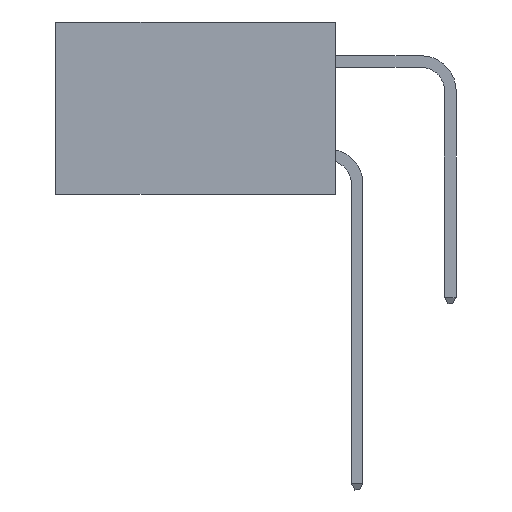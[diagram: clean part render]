
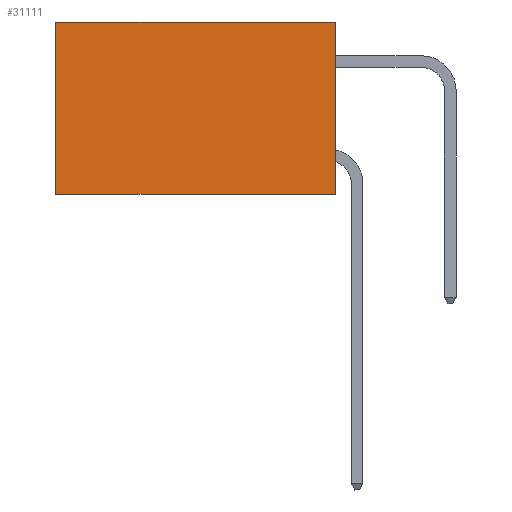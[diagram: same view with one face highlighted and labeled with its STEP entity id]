
A CAD part, left-side view. The second image highlights one B-rep face of the part: STEP entity #31111.
In plain terms, the highlighted planar face has unit normal (-1, 0, 0).
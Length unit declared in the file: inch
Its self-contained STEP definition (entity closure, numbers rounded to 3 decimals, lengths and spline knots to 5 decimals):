
#337 = EDGE_LOOP ( 'NONE', ( #29515, #32129, #18010, #15075 ) ) ;
#3895 = EDGE_CURVE ( 'NONE', #24921, #23185, #25871, .T. ) ;
#4324 = EDGE_CURVE ( 'NONE', #21597, #24921, #25667, .T. ) ;
#5169 = AXIS2_PLACEMENT_3D ( 'NONE', #15169, #25221, #10219 ) ;
#5668 = VERTEX_POINT ( 'NONE', #9489 ) ;
#9489 = CARTESIAN_POINT ( 'NONE',  ( 0.2875, 0.6, 0. ) ) ;
#9986 = FACE_OUTER_BOUND ( 'NONE', #337, .T. ) ;
#10219 = DIRECTION ( 'NONE',  ( 0., 0., -1. ) ) ;
#10356 = DIRECTION ( 'NONE',  ( 0., 0., -1. ) ) ;
#10673 = VECTOR ( 'NONE', #10356, 39.37008 ) ;
#11401 = CARTESIAN_POINT ( 'NONE',  ( 0.2875, 0., 0. ) ) ;
#12891 = CARTESIAN_POINT ( 'NONE',  ( 0.2875, 0.6, 0. ) ) ;
#15075 = ORIENTED_EDGE ( 'NONE', *, *, #28272, .T. ) ;
#15169 = CARTESIAN_POINT ( 'NONE',  ( 0.2875, 0., 0. ) ) ;
#17122 = DIRECTION ( 'NONE',  ( 0., 1., 0. ) ) ;
#18010 = ORIENTED_EDGE ( 'NONE', *, *, #4324, .F. ) ;
#18262 = VECTOR ( 'NONE', #31978, 39.37008 ) ;
#20054 = CARTESIAN_POINT ( 'NONE',  ( 0.2875, 0., -0.37 ) ) ;
#21597 = VERTEX_POINT ( 'NONE', #23201 ) ;
#22123 = CARTESIAN_POINT ( 'NONE',  ( 0.2875, 0.6, -0.37 ) ) ;
#22314 = CARTESIAN_POINT ( 'NONE',  ( 0.2875, 0., -0.37 ) ) ;
#22749 = PLANE ( 'NONE',  #5169 ) ;
#23185 = VERTEX_POINT ( 'NONE', #22123 ) ;
#23201 = CARTESIAN_POINT ( 'NONE',  ( 0.2875, 0., 0. ) ) ;
#23402 = EDGE_CURVE ( 'NONE', #5668, #23185, #30554, .T. ) ;
#24921 = VERTEX_POINT ( 'NONE', #22314 ) ;
#25123 = VECTOR ( 'NONE', #17122, 39.37008 ) ;
#25221 = DIRECTION ( 'NONE',  ( 1., 0., 0. ) ) ;
#25667 = LINE ( 'NONE', #29577, #18262 ) ;
#25871 = LINE ( 'NONE', #20054, #25123 ) ;
#28272 = EDGE_CURVE ( 'NONE', #21597, #5668, #28339, .T. ) ;
#28339 = LINE ( 'NONE', #11401, #29118 ) ;
#28848 = DIRECTION ( 'NONE',  ( 0., 1., 0. ) ) ;
#29118 = VECTOR ( 'NONE', #28848, 39.37008 ) ;
#29515 = ORIENTED_EDGE ( 'NONE', *, *, #23402, .T. ) ;
#29577 = CARTESIAN_POINT ( 'NONE',  ( 0.2875, 0., 0. ) ) ;
#30554 = LINE ( 'NONE', #12891, #10673 ) ;
#31111 = ADVANCED_FACE ( 'NONE', ( #9986 ), #22749, .F. ) ;
#31978 = DIRECTION ( 'NONE',  ( 0., 0., -1. ) ) ;
#32129 = ORIENTED_EDGE ( 'NONE', *, *, #3895, .F. ) ;
